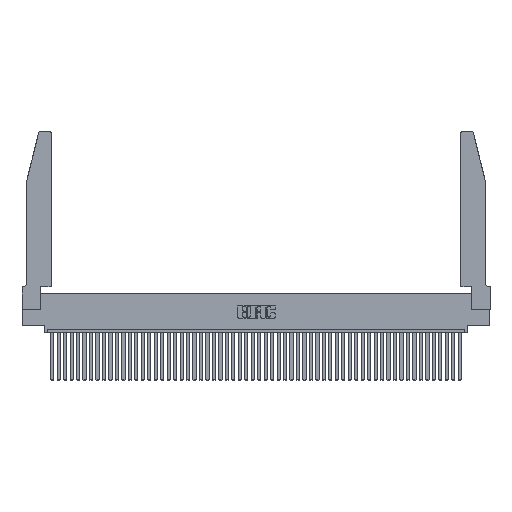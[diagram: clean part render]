
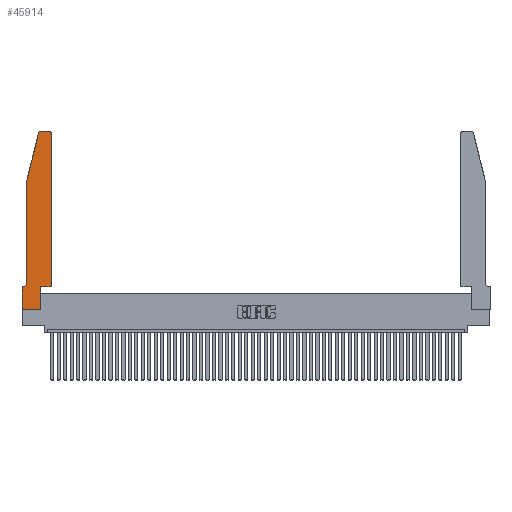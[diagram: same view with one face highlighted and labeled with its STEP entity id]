
A CAD part, top view. The second image highlights one B-rep face of the part: STEP entity #45914.
In plain terms, the highlighted planar face has unit normal (0, 0, 1).
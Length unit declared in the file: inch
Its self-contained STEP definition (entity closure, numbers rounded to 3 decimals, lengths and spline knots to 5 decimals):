
#2259 = CARTESIAN_POINT ( 'NONE',  ( 0.284, 2.72, 0.37 ) ) ;
#2509 = VECTOR ( 'NONE', #18540, 39.37008 ) ;
#3049 = LINE ( 'NONE', #36376, #19818 ) ;
#4391 = EDGE_CURVE ( 'NONE', #31119, #15733, #6203, .T. ) ;
#5555 = CARTESIAN_POINT ( 'NONE',  ( 0.0755, 2., 0.37 ) ) ;
#6203 = CIRCLE ( 'NONE', #23849, 0.03 ) ;
#6229 = EDGE_CURVE ( 'NONE', #26220, #47042, #30492, .T. ) ;
#6859 = DIRECTION ( 'NONE',  ( 1., 0., 0. ) ) ;
#7455 = EDGE_CURVE ( 'NONE', #15733, #24955, #33506, .T. ) ;
#8285 = PLANE ( 'NONE',  #23276 ) ;
#8612 = CARTESIAN_POINT ( 'NONE',  ( 0.2865, 0.35, 0.37 ) ) ;
#8830 = VERTEX_POINT ( 'NONE', #39960 ) ;
#9002 = CARTESIAN_POINT ( 'NONE',  ( 0.0055, 0.42, 0.37 ) ) ;
#9373 = EDGE_CURVE ( 'NONE', #47042, #24021, #47057, .T. ) ;
#9751 = EDGE_CURVE ( 'NONE', #24955, #48766, #28966, .T. ) ;
#9852 = DIRECTION ( 'NONE',  ( 0., 1., 0. ) ) ;
#9865 = CARTESIAN_POINT ( 'NONE',  ( 0.2605, 2.75, 0.37 ) ) ;
#9977 = VECTOR ( 'NONE', #16750, 39.37008 ) ;
#10049 = ORIENTED_EDGE ( 'NONE', *, *, #10403, .T. ) ;
#10069 = VERTEX_POINT ( 'NONE', #18364 ) ;
#10403 = EDGE_CURVE ( 'NONE', #24021, #37825, #27081, .T. ) ;
#10648 = CARTESIAN_POINT ( 'NONE',  ( 0., 0., 0.37 ) ) ;
#11013 = EDGE_CURVE ( 'NONE', #34831, #26220, #30036, .T. ) ;
#11055 = ORIENTED_EDGE ( 'NONE', *, *, #18095, .T. ) ;
#12011 = CARTESIAN_POINT ( 'NONE',  ( 0.4505, 2.72, 0.37 ) ) ;
#12038 = DIRECTION ( 'NONE',  ( 1., 0., 0. ) ) ;
#12100 = CARTESIAN_POINT ( 'NONE',  ( 0., 0.35, 0.37 ) ) ;
#12388 = VERTEX_POINT ( 'NONE', #5555 ) ;
#13807 = ORIENTED_EDGE ( 'NONE', *, *, #4391, .T. ) ;
#13860 = CARTESIAN_POINT ( 'NONE',  ( 0.4205, 2.75, 0.37 ) ) ;
#14654 = DIRECTION ( 'NONE',  ( 0., 0., 1. ) ) ;
#15067 = ORIENTED_EDGE ( 'NONE', *, *, #11013, .T. ) ;
#15078 = LINE ( 'NONE', #41358, #2509 ) ;
#15733 = VERTEX_POINT ( 'NONE', #13860 ) ;
#15741 = CARTESIAN_POINT ( 'NONE',  ( 0., 0.35, 0.37 ) ) ;
#16073 = ORIENTED_EDGE ( 'NONE', *, *, #6229, .T. ) ;
#16750 = DIRECTION ( 'NONE',  ( 0., -1., 0. ) ) ;
#16874 = DIRECTION ( 'NONE',  ( -1., 0., 0. ) ) ;
#18095 = EDGE_CURVE ( 'NONE', #12388, #10069, #29667, .T. ) ;
#18364 = CARTESIAN_POINT ( 'NONE',  ( 0.0755, 0.42, 0.37 ) ) ;
#18540 = DIRECTION ( 'NONE',  ( -0.239, -0.971, 0. ) ) ;
#19122 = AXIS2_PLACEMENT_3D ( 'NONE', #2259, #28994, #48030 ) ;
#19226 = ORIENTED_EDGE ( 'NONE', *, *, #37667, .T. ) ;
#19384 = EDGE_CURVE ( 'NONE', #10069, #34831, #32560, .T. ) ;
#19474 = DIRECTION ( 'NONE',  ( -1., 0., 0. ) ) ;
#19641 = CARTESIAN_POINT ( 'NONE',  ( 0.0755, 0.35, 0.37 ) ) ;
#19818 = VECTOR ( 'NONE', #9852, 39.37008 ) ;
#21257 = CARTESIAN_POINT ( 'NONE',  ( 0.284, 2.75, 0.37 ) ) ;
#22089 = FACE_OUTER_BOUND ( 'NONE', #29928, .T. ) ;
#22282 = DIRECTION ( 'NONE',  ( 0., -1., 0. ) ) ;
#22419 = DIRECTION ( 'NONE',  ( 1., 0., 0. ) ) ;
#23276 = AXIS2_PLACEMENT_3D ( 'NONE', #12100, #14654, #22419 ) ;
#23849 = AXIS2_PLACEMENT_3D ( 'NONE', #26038, #41890, #6859 ) ;
#24021 = VERTEX_POINT ( 'NONE', #35398 ) ;
#24775 = ORIENTED_EDGE ( 'NONE', *, *, #40654, .T. ) ;
#24877 = AXIS2_PLACEMENT_3D ( 'NONE', #9002, #44199, #16874 ) ;
#24955 = VERTEX_POINT ( 'NONE', #21257 ) ;
#26006 = VECTOR ( 'NONE', #12038, 39.37008 ) ;
#26038 = CARTESIAN_POINT ( 'NONE',  ( 0.4205, 2.72, 0.37 ) ) ;
#26220 = VERTEX_POINT ( 'NONE', #15741 ) ;
#27081 = LINE ( 'NONE', #8612, #40427 ) ;
#27214 = ORIENTED_EDGE ( 'NONE', *, *, #43761, .T. ) ;
#27459 = LINE ( 'NONE', #32445, #45563 ) ;
#28139 = DIRECTION ( 'NONE',  ( 0., 1., 0. ) ) ;
#28558 = CARTESIAN_POINT ( 'NONE',  ( 0., 0., 0.37 ) ) ;
#28815 = VECTOR ( 'NONE', #19474, 39.37008 ) ;
#28966 = CIRCLE ( 'NONE', #19122, 0.03 ) ;
#28994 = DIRECTION ( 'NONE',  ( 0., 0., 1. ) ) ;
#29425 = CARTESIAN_POINT ( 'NONE',  ( 0.0055, 0.35, 0.37 ) ) ;
#29667 = LINE ( 'NONE', #41550, #47087 ) ;
#29928 = EDGE_LOOP ( 'NONE', ( #32644, #42958, #27214, #11055, #34526, #15067, #16073, #32590, #10049, #24775, #19226, #13807 ) ) ;
#30036 = LINE ( 'NONE', #19641, #28815 ) ;
#30492 = LINE ( 'NONE', #28558, #9977 ) ;
#31119 = VERTEX_POINT ( 'NONE', #12011 ) ;
#32445 = CARTESIAN_POINT ( 'NONE',  ( 0.4505, 0.35, 0.37 ) ) ;
#32560 = CIRCLE ( 'NONE', #24877, 0.07 ) ;
#32590 = ORIENTED_EDGE ( 'NONE', *, *, #9373, .T. ) ;
#32644 = ORIENTED_EDGE ( 'NONE', *, *, #7455, .T. ) ;
#33506 = LINE ( 'NONE', #9865, #48525 ) ;
#34526 = ORIENTED_EDGE ( 'NONE', *, *, #19384, .T. ) ;
#34831 = VERTEX_POINT ( 'NONE', #29425 ) ;
#35398 = CARTESIAN_POINT ( 'NONE',  ( 0.2865, 0., 0.37 ) ) ;
#36376 = CARTESIAN_POINT ( 'NONE',  ( 0.4505, 0.35, 0.37 ) ) ;
#37667 = EDGE_CURVE ( 'NONE', #8830, #31119, #3049, .T. ) ;
#37825 = VERTEX_POINT ( 'NONE', #48777 ) ;
#39960 = CARTESIAN_POINT ( 'NONE',  ( 0.4505, 0.35, 0.37 ) ) ;
#40427 = VECTOR ( 'NONE', #28139, 39.37008 ) ;
#40654 = EDGE_CURVE ( 'NONE', #37825, #8830, #27459, .T. ) ;
#41358 = CARTESIAN_POINT ( 'NONE',  ( 0.0755, 2., 0.37 ) ) ;
#41382 = DIRECTION ( 'NONE',  ( 1., 0., 0. ) ) ;
#41550 = CARTESIAN_POINT ( 'NONE',  ( 0.0755, 2., 0.37 ) ) ;
#41890 = DIRECTION ( 'NONE',  ( 0., 0., 1. ) ) ;
#42958 = ORIENTED_EDGE ( 'NONE', *, *, #9751, .T. ) ;
#43092 = CARTESIAN_POINT ( 'NONE',  ( 0., 0., 0.37 ) ) ;
#43761 = EDGE_CURVE ( 'NONE', #48766, #12388, #15078, .T. ) ;
#44199 = DIRECTION ( 'NONE',  ( 0., 0., -1. ) ) ;
#45563 = VECTOR ( 'NONE', #41382, 39.37008 ) ;
#45914 = ADVANCED_FACE ( 'NONE', ( #22089 ), #8285, .T. ) ;
#47042 = VERTEX_POINT ( 'NONE', #10648 ) ;
#47057 = LINE ( 'NONE', #43092, #26006 ) ;
#47087 = VECTOR ( 'NONE', #22282, 39.37008 ) ;
#48030 = DIRECTION ( 'NONE',  ( 1., 0., 0. ) ) ;
#48449 = DIRECTION ( 'NONE',  ( -1., 0., 0. ) ) ;
#48525 = VECTOR ( 'NONE', #48449, 39.37008 ) ;
#48766 = VERTEX_POINT ( 'NONE', #48925 ) ;
#48777 = CARTESIAN_POINT ( 'NONE',  ( 0.2865, 0.35, 0.37 ) ) ;
#48925 = CARTESIAN_POINT ( 'NONE',  ( 0.25487, 2.72718, 0.37 ) ) ;
